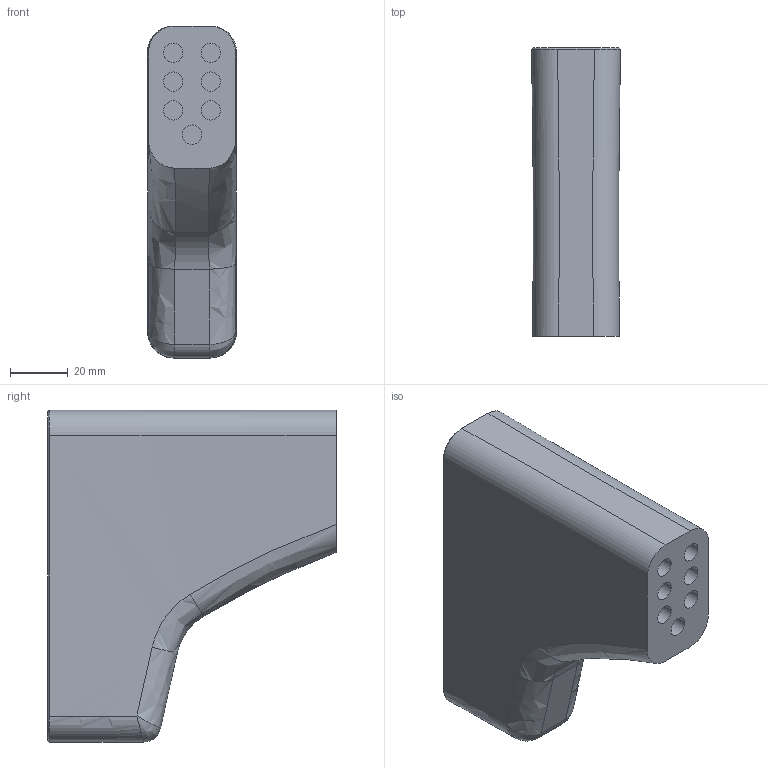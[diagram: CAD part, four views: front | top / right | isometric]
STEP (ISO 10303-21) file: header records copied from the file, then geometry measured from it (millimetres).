
FILE_DESCRIPTION(/* description */ (''),/* implementation_level */ '2;1');
FILE_NAME(/* name */ 'Butt Half.step',/* time_stamp */ '2021-07-28T09:04:16-04:00',/* author */ (''),/* organization */ (''),/* preprocessor_version */ 'ST-DEVELOPER v18.1',/* originating_system */ 'Autodesk Translation Framework v10.9.0.1377',/* authorisation */ '');
FILE_SCHEMA (('AUTOMOTIVE_DESIGN { 1 0 10303 214 3 1 1 }'));
Length unit declared in the file: millimetre
Products named in the file (1): Butt Half
Bounding box: 30.77 x 100 x 115 mm (x, y, z)
Volume: 134565.6 mm3; surface area: 43111.1 mm2
Topology: 1 solids, 1 shells, 132 faces, 297 edges, 172 vertices
Faces by surface type: bspline 42, plane 36, cylinder 32, torus 16, cone 6
Full cylindrical faces by diameter (mm): 4 x2, 6.7 x7
Entity records: 5858 total; most frequent: CARTESIAN_POINT 3109, ORIENTED_EDGE 578, DIRECTION 513, EDGE_CURVE 289, AXIS2_PLACEMENT_3D 207, VERTEX_POINT 172, EDGE_LOOP 149, FACE_OUTER_BOUND 132
